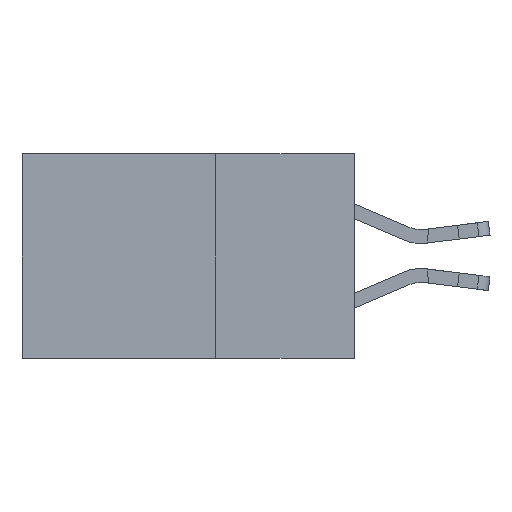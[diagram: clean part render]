
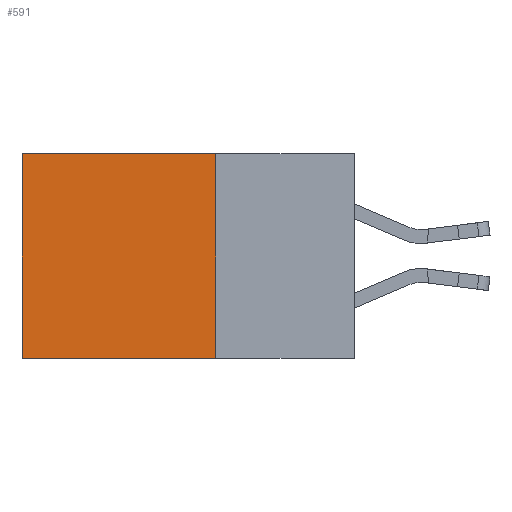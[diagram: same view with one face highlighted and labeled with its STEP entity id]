
A CAD part, left-side view. The second image highlights one B-rep face of the part: STEP entity #591.
In plain terms, the highlighted planar face has unit normal (-1, 0, 0).
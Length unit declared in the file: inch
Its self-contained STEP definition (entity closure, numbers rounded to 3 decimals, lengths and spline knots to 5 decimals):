
#468 = LINE ( 'NONE', #14059, #2605 ) ;
#591 = ADVANCED_FACE ( 'NONE', ( #4161 ), #8648, .F. ) ;
#844 = ORIENTED_EDGE ( 'NONE', *, *, #4312, .F. ) ;
#1952 = DIRECTION ( 'NONE',  ( 0., 0., -1. ) ) ;
#2023 = DIRECTION ( 'NONE',  ( 1., 0., 0. ) ) ;
#2365 = DIRECTION ( 'NONE',  ( 0., 1., 0. ) ) ;
#2605 = VECTOR ( 'NONE', #10838, 39.37008 ) ;
#3014 = VECTOR ( 'NONE', #11833, 39.37008 ) ;
#3267 = VERTEX_POINT ( 'NONE', #7800 ) ;
#3892 = ORIENTED_EDGE ( 'NONE', *, *, #4704, .T. ) ;
#4026 = CARTESIAN_POINT ( 'NONE',  ( 0.2615, 0.6, -0.37 ) ) ;
#4161 = FACE_OUTER_BOUND ( 'NONE', #14270, .T. ) ;
#4273 = CARTESIAN_POINT ( 'NONE',  ( 0.2615, 0.6, -0.37 ) ) ;
#4312 = EDGE_CURVE ( 'NONE', #9492, #12004, #12379, .T. ) ;
#4430 = CARTESIAN_POINT ( 'NONE',  ( 0.2615, 0.6, 0. ) ) ;
#4704 = EDGE_CURVE ( 'NONE', #10487, #12004, #10874, .T. ) ;
#6122 = VECTOR ( 'NONE', #2365, 39.37008 ) ;
#6400 = DIRECTION ( 'NONE',  ( 0., 0., -1. ) ) ;
#6707 = ORIENTED_EDGE ( 'NONE', *, *, #13258, .T. ) ;
#7800 = CARTESIAN_POINT ( 'NONE',  ( 0.2615, 0.25, 0. ) ) ;
#8256 = AXIS2_PLACEMENT_3D ( 'NONE', #13140, #2023, #1952 ) ;
#8286 = VECTOR ( 'NONE', #6400, 39.37008 ) ;
#8648 = PLANE ( 'NONE',  #8256 ) ;
#9062 = ORIENTED_EDGE ( 'NONE', *, *, #9170, .F. ) ;
#9170 = EDGE_CURVE ( 'NONE', #3267, #9492, #13079, .T. ) ;
#9492 = VERTEX_POINT ( 'NONE', #13656 ) ;
#10487 = VERTEX_POINT ( 'NONE', #4430 ) ;
#10838 = DIRECTION ( 'NONE',  ( 0., 1., 0. ) ) ;
#10874 = LINE ( 'NONE', #4026, #8286 ) ;
#11833 = DIRECTION ( 'NONE',  ( 0., 0., -1. ) ) ;
#12004 = VERTEX_POINT ( 'NONE', #4273 ) ;
#12379 = LINE ( 'NONE', #12525, #6122 ) ;
#12525 = CARTESIAN_POINT ( 'NONE',  ( 0.2615, 0.25, -0.37 ) ) ;
#12809 = CARTESIAN_POINT ( 'NONE',  ( 0.2615, 0.25, -0.37 ) ) ;
#13079 = LINE ( 'NONE', #12809, #3014 ) ;
#13140 = CARTESIAN_POINT ( 'NONE',  ( 0.2615, 0.25, -0.37 ) ) ;
#13258 = EDGE_CURVE ( 'NONE', #3267, #10487, #468, .T. ) ;
#13656 = CARTESIAN_POINT ( 'NONE',  ( 0.2615, 0.25, -0.37 ) ) ;
#14059 = CARTESIAN_POINT ( 'NONE',  ( 0.2615, 0.25, 0. ) ) ;
#14270 = EDGE_LOOP ( 'NONE', ( #3892, #844, #9062, #6707 ) ) ;
